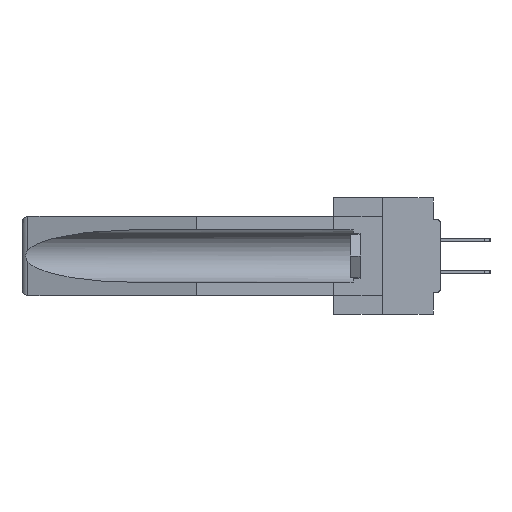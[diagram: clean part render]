
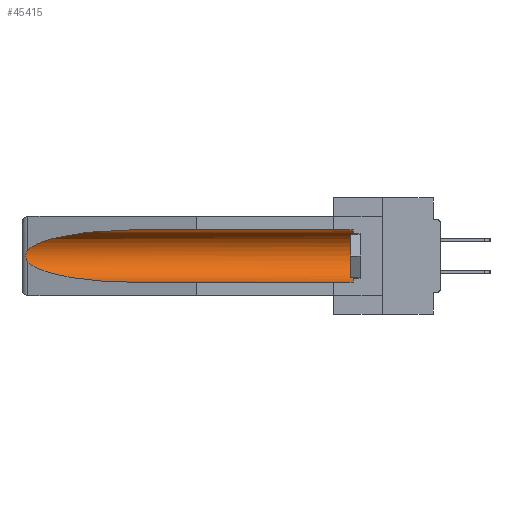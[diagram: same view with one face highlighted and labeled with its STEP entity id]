
A CAD part, left-side view. The second image highlights one B-rep face of the part: STEP entity #45415.
In plain terms, the highlighted cylindrical face has radius 2.857 mm (diameter 5.715 mm), a partial arc.
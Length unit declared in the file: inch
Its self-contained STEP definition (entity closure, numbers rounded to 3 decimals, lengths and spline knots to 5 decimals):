
#336 = CARTESIAN_POINT ( 'NONE',  ( 0.26537, 1.52718, -0.14972 ) ) ;
#1044 = EDGE_LOOP ( 'NONE', ( #37928, #33341, #4189, #13608, #20810, #3350 ) ) ;
#2202 =( BOUNDED_CURVE ( )  B_SPLINE_CURVE ( 3, ( #29784, #29461, #8159, #25981 ),
 .UNSPECIFIED., .F., .F. ) 
 B_SPLINE_CURVE_WITH_KNOTS ( ( 4, 4 ),
 ( 0.1948, 1.5708 ),
 .UNSPECIFIED. ) 
 CURVE ( )  GEOMETRIC_REPRESENTATION_ITEM ( )  RATIONAL_B_SPLINE_CURVE ( ( 1., 0.848, 0.848, 1. ) ) 
 REPRESENTATION_ITEM ( '' )  );
#3047 = DIRECTION ( 'NONE',  ( 0., 1., 0. ) ) ;
#3350 = ORIENTED_EDGE ( 'NONE', *, *, #10622, .T. ) ;
#3989 = CARTESIAN_POINT ( 'NONE',  ( 0.26537, 1.52718, -0.14972 ) ) ;
#4189 = ORIENTED_EDGE ( 'NONE', *, *, #25416, .T. ) ;
#4632 = DIRECTION ( 'NONE',  ( 0., 0., 1. ) ) ;
#6234 = EDGE_CURVE ( 'NONE', #10712, #42733, #19020, .T. ) ;
#8159 = CARTESIAN_POINT ( 'NONE',  ( 0.21114, 1.30732, -0.284 ) ) ;
#8283 = CARTESIAN_POINT ( 'NONE',  ( 0.26537, 1.52718, -0.19328 ) ) ;
#9202 = AXIS2_PLACEMENT_3D ( 'NONE', #24157, #42137, #20489 ) ;
#9398 = CYLINDRICAL_SURFACE ( 'NONE', #24022, 0.1125 ) ;
#10622 = EDGE_CURVE ( 'NONE', #22583, #10712, #41527, .T. ) ;
#10645 = CARTESIAN_POINT ( 'NONE',  ( 0.155, -0.30754, -0.284 ) ) ;
#10712 = VERTEX_POINT ( 'NONE', #24972 ) ;
#11075 = CARTESIAN_POINT ( 'NONE',  ( 0.26537, 1.52718, -0.19328 ) ) ;
#11197 = EDGE_CURVE ( 'NONE', #18139, #22583, #32394, .T. ) ;
#11555 = CARTESIAN_POINT ( 'NONE',  ( 0.2675, 1.53308, -0.17534 ) ) ;
#12817 = VERTEX_POINT ( 'NONE', #22550 ) ;
#13231 = CARTESIAN_POINT ( 'NONE',  ( 0.155, -0.30754, -0.1715 ) ) ;
#13303 = FACE_OUTER_BOUND ( 'NONE', #1044, .T. ) ;
#13608 = ORIENTED_EDGE ( 'NONE', *, *, #44248, .F. ) ;
#14532 = CARTESIAN_POINT ( 'NONE',  ( 0.155, 0.126, -0.284 ) ) ;
#14553 = CARTESIAN_POINT ( 'NONE',  ( 0.26654, 1.53092, -0.15636 ) ) ;
#16795 = VERTEX_POINT ( 'NONE', #8283 ) ;
#17036 = DIRECTION ( 'NONE',  ( 0., 1., 0. ) ) ;
#18139 = VERTEX_POINT ( 'NONE', #14532 ) ;
#18232 = CARTESIAN_POINT ( 'NONE',  ( 0.25451, 1.48313, -0.09465 ) ) ;
#18373 = CARTESIAN_POINT ( 'NONE',  ( 0.155, 1.07973, -0.059 ) ) ;
#18831 = CARTESIAN_POINT ( 'NONE',  ( 0.2673, 1.53269, -0.17917 ) ) ;
#19020 =( BOUNDED_CURVE ( )  B_SPLINE_CURVE ( 3, ( #18373, #25477, #18232, #336 ),
 .UNSPECIFIED., .F., .F. ) 
 B_SPLINE_CURVE_WITH_KNOTS ( ( 4, 4 ),
 ( 4.71239, 6.08839 ),
 .UNSPECIFIED. ) 
 CURVE ( )  GEOMETRIC_REPRESENTATION_ITEM ( )  RATIONAL_B_SPLINE_CURVE ( ( 1., 0.848, 0.848, 1. ) ) 
 REPRESENTATION_ITEM ( '' )  );
#19196 = CARTESIAN_POINT ( 'NONE',  ( 0.155, 0.126, -0.059 ) ) ;
#20489 = DIRECTION ( 'NONE',  ( 0., 0., 1. ) ) ;
#20810 = ORIENTED_EDGE ( 'NONE', *, *, #11197, .T. ) ;
#21818 = CARTESIAN_POINT ( 'NONE',  ( 0.2673, 1.5327, -0.16383 ) ) ;
#21973 = CARTESIAN_POINT ( 'NONE',  ( 0.2675, 1.53308, -0.16763 ) ) ;
#22550 = CARTESIAN_POINT ( 'NONE',  ( 0.155, 1.07973, -0.284 ) ) ;
#22583 = VERTEX_POINT ( 'NONE', #19196 ) ;
#23452 = VECTOR ( 'NONE', #3047, 39.37008 ) ;
#24022 = AXIS2_PLACEMENT_3D ( 'NONE', #13231, #17036, #4632 ) ;
#24157 = CARTESIAN_POINT ( 'NONE',  ( 0.155, 0.126, -0.1715 ) ) ;
#24972 = CARTESIAN_POINT ( 'NONE',  ( 0.155, 1.07973, -0.059 ) ) ;
#25416 = EDGE_CURVE ( 'NONE', #16795, #12817, #2202, .T. ) ;
#25477 = CARTESIAN_POINT ( 'NONE',  ( 0.21114, 1.30732, -0.059 ) ) ;
#25981 = CARTESIAN_POINT ( 'NONE',  ( 0.155, 1.07973, -0.284 ) ) ;
#26067 = CARTESIAN_POINT ( 'NONE',  ( 0.26655, 1.53094, -0.18657 ) ) ;
#26476 = EDGE_CURVE ( 'NONE', #42733, #16795, #27941, .T. ) ;
#27941 = B_SPLINE_CURVE_WITH_KNOTS ( 'NONE', 3,
 ( #43593, #32689, #14553, #21818, #21973, #11555, #18831, #26067, #33337, #11075 ),
 .UNSPECIFIED., .F., .F.,
 ( 4, 2, 2, 2, 4 ),
 ( 0., 0.00029, 0.00058, 0.00087, 0.00117 ),
 .UNSPECIFIED. ) ;
#29461 = CARTESIAN_POINT ( 'NONE',  ( 0.25451, 1.48313, -0.24835 ) ) ;
#29784 = CARTESIAN_POINT ( 'NONE',  ( 0.26537, 1.52718, -0.19328 ) ) ;
#30604 = LINE ( 'NONE', #10645, #35025 ) ;
#31779 = DIRECTION ( 'NONE',  ( 0., 1., 0. ) ) ;
#32394 = CIRCLE ( 'NONE', #9202, 0.1125 ) ;
#32689 = CARTESIAN_POINT ( 'NONE',  ( 0.26597, 1.52961, -0.15275 ) ) ;
#33337 = CARTESIAN_POINT ( 'NONE',  ( 0.26597, 1.5296, -0.19026 ) ) ;
#33341 = ORIENTED_EDGE ( 'NONE', *, *, #26476, .T. ) ;
#35025 = VECTOR ( 'NONE', #31779, 39.37008 ) ;
#37928 = ORIENTED_EDGE ( 'NONE', *, *, #6234, .T. ) ;
#41527 = LINE ( 'NONE', #46158, #23452 ) ;
#42137 = DIRECTION ( 'NONE',  ( 0., -1., 0. ) ) ;
#42733 = VERTEX_POINT ( 'NONE', #3989 ) ;
#43593 = CARTESIAN_POINT ( 'NONE',  ( 0.26537, 1.52718, -0.14972 ) ) ;
#44248 = EDGE_CURVE ( 'NONE', #18139, #12817, #30604, .T. ) ;
#45415 = ADVANCED_FACE ( 'NONE', ( #13303 ), #9398, .F. ) ;
#46158 = CARTESIAN_POINT ( 'NONE',  ( 0.155, -0.30754, -0.059 ) ) ;
